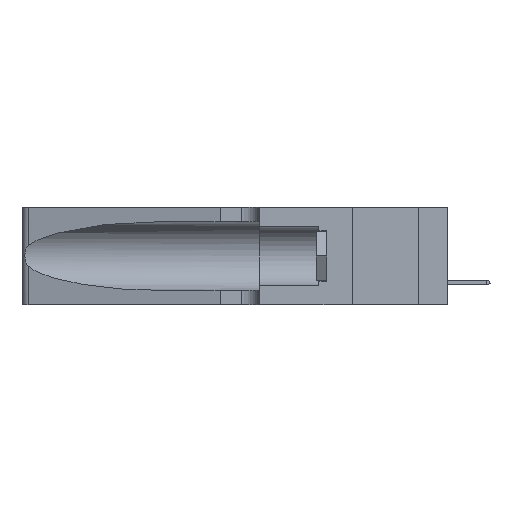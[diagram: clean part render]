
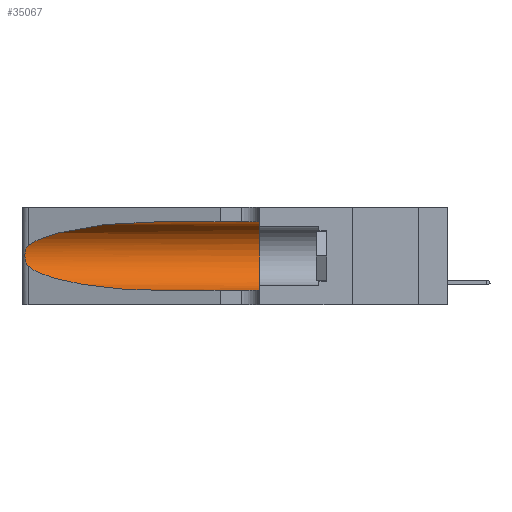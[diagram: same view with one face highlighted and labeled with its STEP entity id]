
A CAD part, left-side view. The second image highlights one B-rep face of the part: STEP entity #35067.
In plain terms, the highlighted cylindrical face has radius 3.308 mm (diameter 6.617 mm), a partial arc.
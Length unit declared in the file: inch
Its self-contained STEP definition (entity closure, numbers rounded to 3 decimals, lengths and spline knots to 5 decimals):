
#179 = CARTESIAN_POINT ( 'NONE',  ( 0.1305, 1.61858, 0.185 ) ) ;
#525 = CYLINDRICAL_SURFACE ( 'NONE', #31165, 0.13025 ) ;
#607 = CARTESIAN_POINT ( 'NONE',  ( 0.18966, 0.96281, 0.31525 ) ) ;
#1077 = CARTESIAN_POINT ( 'NONE',  ( 0.2373, 1.15595, 0.08982 ) ) ;
#1448 = ORIENTED_EDGE ( 'NONE', *, *, #9204, .T. ) ;
#2532 = CARTESIAN_POINT ( 'NONE',  ( 0.1305, 0.72297, 0.31525 ) ) ;
#2887 = VECTOR ( 'NONE', #9834, 39.37008 ) ;
#4868 = CARTESIAN_POINT ( 'NONE',  ( 0.1305, 0.72297, 0.31525 ) ) ;
#5257 =( BOUNDED_CURVE ( )  B_SPLINE_CURVE ( 3, ( #2532, #607, #26940, #24588 ),
 .UNSPECIFIED., .F., .F. ) 
 B_SPLINE_CURVE_WITH_KNOTS ( ( 4, 4 ),
 ( 1.5708, 2.84003 ),
 .UNSPECIFIED. ) 
 CURVE ( )  GEOMETRIC_REPRESENTATION_ITEM ( )  RATIONAL_B_SPLINE_CURVE ( ( 1., 0.87, 0.87, 1. ) ) 
 REPRESENTATION_ITEM ( '' )  );
#5643 = VERTEX_POINT ( 'NONE', #36268 ) ;
#6648 = CARTESIAN_POINT ( 'NONE',  ( 0.18966, 0.96281, 0.05475 ) ) ;
#6772 = CARTESIAN_POINT ( 'NONE',  ( 0.25487, 1.22718, 0.14631 ) ) ;
#6813 = FACE_OUTER_BOUND ( 'NONE', #11116, .T. ) ;
#8481 = CARTESIAN_POINT ( 'NONE',  ( 0.26018, 1.23835, 0.19895 ) ) ;
#9204 = EDGE_CURVE ( 'NONE', #25928, #32961, #10652, .T. ) ;
#9580 = CARTESIAN_POINT ( 'NONE',  ( 0.25639, 1.23184, 0.21858 ) ) ;
#9834 = DIRECTION ( 'NONE',  ( 0., -1., 0. ) ) ;
#10652 = B_SPLINE_CURVE_WITH_KNOTS ( 'NONE', 3,
 ( #23825, #14634, #9580, #22462, #39429, #8481, #11059, #11574, #36143, #36012, #17412, #20669, #39159, #33274 ),
 .UNSPECIFIED., .F., .F.,
 ( 4, 2, 2, 2, 2, 2, 4 ),
 ( 0., 0.00027, 0.00053, 0.00107, 0.0016, 0.00187, 0.00214 ),
 .UNSPECIFIED. ) ;
#11059 = CARTESIAN_POINT ( 'NONE',  ( 0.26075, 1.23896, 0.19203 ) ) ;
#11116 = EDGE_LOOP ( 'NONE', ( #13305, #1448, #34091, #21802, #36530, #18456 ) ) ;
#11574 = CARTESIAN_POINT ( 'NONE',  ( 0.26075, 1.23896, 0.178 ) ) ;
#12935 = CIRCLE ( 'NONE', #18572, 0.13025 ) ;
#13305 = ORIENTED_EDGE ( 'NONE', *, *, #14533, .T. ) ;
#13815 = VERTEX_POINT ( 'NONE', #37542 ) ;
#14533 = EDGE_CURVE ( 'NONE', #27355, #25928, #5257, .T. ) ;
#14634 = CARTESIAN_POINT ( 'NONE',  ( 0.25555, 1.22994, 0.2215 ) ) ;
#16795 = EDGE_CURVE ( 'NONE', #5643, #35118, #12935, .T. ) ;
#17412 = CARTESIAN_POINT ( 'NONE',  ( 0.25789, 1.23486, 0.15765 ) ) ;
#18338 = LINE ( 'NONE', #37125, #2887 ) ;
#18456 = ORIENTED_EDGE ( 'NONE', *, *, #38733, .F. ) ;
#18572 = AXIS2_PLACEMENT_3D ( 'NONE', #34405, #37550, #25421 ) ;
#18699 = CARTESIAN_POINT ( 'NONE',  ( 0.1305, 0.35, 0.05475 ) ) ;
#19521 = CARTESIAN_POINT ( 'NONE',  ( 0.25487, 1.22718, 0.22369 ) ) ;
#20669 = CARTESIAN_POINT ( 'NONE',  ( 0.25639, 1.23186, 0.15144 ) ) ;
#21057 = EDGE_CURVE ( 'NONE', #32961, #13815, #26811, .T. ) ;
#21390 = VECTOR ( 'NONE', #36958, 39.37008 ) ;
#21802 = ORIENTED_EDGE ( 'NONE', *, *, #33826, .T. ) ;
#21944 = DIRECTION ( 'NONE',  ( 0., 0., -1. ) ) ;
#22462 = CARTESIAN_POINT ( 'NONE',  ( 0.25787, 1.23484, 0.2124 ) ) ;
#23825 = CARTESIAN_POINT ( 'NONE',  ( 0.25487, 1.22718, 0.22369 ) ) ;
#24588 = CARTESIAN_POINT ( 'NONE',  ( 0.25487, 1.22718, 0.22369 ) ) ;
#25421 = DIRECTION ( 'NONE',  ( 0., 0., 1. ) ) ;
#25928 = VERTEX_POINT ( 'NONE', #19521 ) ;
#26811 =( BOUNDED_CURVE ( )  B_SPLINE_CURVE ( 3, ( #6772, #1077, #6648, #28559 ),
 .UNSPECIFIED., .F., .F. ) 
 B_SPLINE_CURVE_WITH_KNOTS ( ( 4, 4 ),
 ( 3.44316, 4.71239 ),
 .UNSPECIFIED. ) 
 CURVE ( )  GEOMETRIC_REPRESENTATION_ITEM ( )  RATIONAL_B_SPLINE_CURVE ( ( 1., 0.87, 0.87, 1. ) ) 
 REPRESENTATION_ITEM ( '' )  );
#26940 = CARTESIAN_POINT ( 'NONE',  ( 0.2373, 1.15595, 0.28018 ) ) ;
#27355 = VERTEX_POINT ( 'NONE', #4868 ) ;
#27587 = CARTESIAN_POINT ( 'NONE',  ( 0.1305, 1.61858, 0.05475 ) ) ;
#28559 = CARTESIAN_POINT ( 'NONE',  ( 0.1305, 0.72297, 0.05475 ) ) ;
#31165 = AXIS2_PLACEMENT_3D ( 'NONE', #179, #37195, #21944 ) ;
#32050 = LINE ( 'NONE', #27587, #21390 ) ;
#32961 = VERTEX_POINT ( 'NONE', #38939 ) ;
#33274 = CARTESIAN_POINT ( 'NONE',  ( 0.25487, 1.22718, 0.14631 ) ) ;
#33826 = EDGE_CURVE ( 'NONE', #13815, #35118, #32050, .T. ) ;
#34091 = ORIENTED_EDGE ( 'NONE', *, *, #21057, .T. ) ;
#34405 = CARTESIAN_POINT ( 'NONE',  ( 0.1305, 0.35, 0.185 ) ) ;
#35067 = ADVANCED_FACE ( 'NONE', ( #6813 ), #525, .F. ) ;
#35118 = VERTEX_POINT ( 'NONE', #18699 ) ;
#36012 = CARTESIAN_POINT ( 'NONE',  ( 0.25856, 1.23593, 0.16098 ) ) ;
#36143 = CARTESIAN_POINT ( 'NONE',  ( 0.26017, 1.23833, 0.17102 ) ) ;
#36268 = CARTESIAN_POINT ( 'NONE',  ( 0.1305, 0.35, 0.31525 ) ) ;
#36530 = ORIENTED_EDGE ( 'NONE', *, *, #16795, .F. ) ;
#36958 = DIRECTION ( 'NONE',  ( 0., -1., 0. ) ) ;
#37125 = CARTESIAN_POINT ( 'NONE',  ( 0.1305, 1.61858, 0.31525 ) ) ;
#37195 = DIRECTION ( 'NONE',  ( 0., -1., 0. ) ) ;
#37542 = CARTESIAN_POINT ( 'NONE',  ( 0.1305, 0.72297, 0.05475 ) ) ;
#37550 = DIRECTION ( 'NONE',  ( 0., 1., 0. ) ) ;
#38733 = EDGE_CURVE ( 'NONE', #27355, #5643, #18338, .T. ) ;
#38939 = CARTESIAN_POINT ( 'NONE',  ( 0.25487, 1.22718, 0.14631 ) ) ;
#39159 = CARTESIAN_POINT ( 'NONE',  ( 0.25555, 1.22993, 0.14849 ) ) ;
#39429 = CARTESIAN_POINT ( 'NONE',  ( 0.25854, 1.2359, 0.20912 ) ) ;
